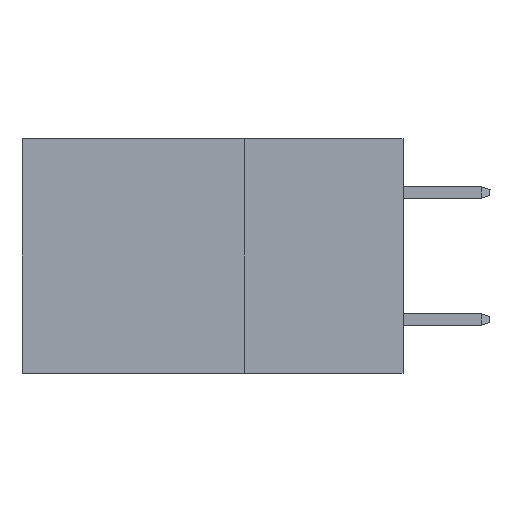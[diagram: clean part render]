
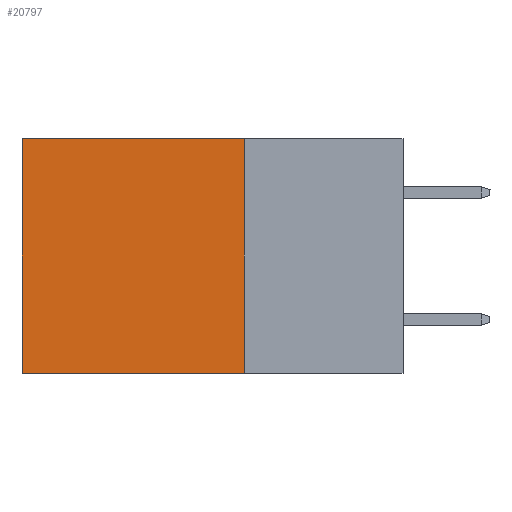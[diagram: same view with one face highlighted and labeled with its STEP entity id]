
A CAD part, left-side view. The second image highlights one B-rep face of the part: STEP entity #20797.
In plain terms, the highlighted planar face has unit normal (-1, 0, 0).
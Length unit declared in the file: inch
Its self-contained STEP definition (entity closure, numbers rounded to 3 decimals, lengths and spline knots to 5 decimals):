
#618 = FACE_OUTER_BOUND ( 'NONE', #32295, .T. ) ;
#2191 = DIRECTION ( 'NONE',  ( 0., 1., 0. ) ) ;
#2203 = CARTESIAN_POINT ( 'NONE',  ( 0.2875, 0.25, 0. ) ) ;
#4341 = ORIENTED_EDGE ( 'NONE', *, *, #25396, .T. ) ;
#4960 = ORIENTED_EDGE ( 'NONE', *, *, #35873, .F. ) ;
#5005 = VECTOR ( 'NONE', #18110, 39.37008 ) ;
#6979 = CARTESIAN_POINT ( 'NONE',  ( 0.2875, 0.6, -0.37 ) ) ;
#7458 = EDGE_CURVE ( 'NONE', #34686, #23279, #25852, .T. ) ;
#7483 = VECTOR ( 'NONE', #35711, 39.37008 ) ;
#10128 = VERTEX_POINT ( 'NONE', #22461 ) ;
#11456 = LINE ( 'NONE', #29577, #19871 ) ;
#14575 = LINE ( 'NONE', #23838, #5005 ) ;
#17661 = VECTOR ( 'NONE', #38244, 39.37008 ) ;
#17678 = CARTESIAN_POINT ( 'NONE',  ( 0.2875, 0.25, -0.37 ) ) ;
#17754 = CARTESIAN_POINT ( 'NONE',  ( 0.2875, 0.25, -0.37 ) ) ;
#17871 = EDGE_CURVE ( 'NONE', #10128, #18480, #11456, .T. ) ;
#18110 = DIRECTION ( 'NONE',  ( 0., 0., -1. ) ) ;
#18480 = VERTEX_POINT ( 'NONE', #24526 ) ;
#19776 = ORIENTED_EDGE ( 'NONE', *, *, #17871, .T. ) ;
#19871 = VECTOR ( 'NONE', #2191, 39.37008 ) ;
#20450 = ORIENTED_EDGE ( 'NONE', *, *, #7458, .F. ) ;
#20797 = ADVANCED_FACE ( 'NONE', ( #618 ), #21661, .F. ) ;
#20887 = DIRECTION ( 'NONE',  ( 1., 0., 0. ) ) ;
#21471 = DIRECTION ( 'NONE',  ( 0., 0., -1. ) ) ;
#21661 = PLANE ( 'NONE',  #32520 ) ;
#22461 = CARTESIAN_POINT ( 'NONE',  ( 0.2875, 0.25, 0. ) ) ;
#23279 = VERTEX_POINT ( 'NONE', #6979 ) ;
#23838 = CARTESIAN_POINT ( 'NONE',  ( 0.2875, 0.6, 0. ) ) ;
#24526 = CARTESIAN_POINT ( 'NONE',  ( 0.2875, 0.6, 0. ) ) ;
#25396 = EDGE_CURVE ( 'NONE', #18480, #23279, #14575, .T. ) ;
#25852 = LINE ( 'NONE', #17754, #7483 ) ;
#28821 = LINE ( 'NONE', #2203, #17661 ) ;
#29577 = CARTESIAN_POINT ( 'NONE',  ( 0.2875, 0.25, 0. ) ) ;
#30176 = CARTESIAN_POINT ( 'NONE',  ( 0.2875, 0.25, 0. ) ) ;
#32295 = EDGE_LOOP ( 'NONE', ( #4341, #20450, #4960, #19776 ) ) ;
#32520 = AXIS2_PLACEMENT_3D ( 'NONE', #30176, #20887, #21471 ) ;
#34686 = VERTEX_POINT ( 'NONE', #17678 ) ;
#35711 = DIRECTION ( 'NONE',  ( 0., 1., 0. ) ) ;
#35873 = EDGE_CURVE ( 'NONE', #10128, #34686, #28821, .T. ) ;
#38244 = DIRECTION ( 'NONE',  ( 0., 0., -1. ) ) ;
